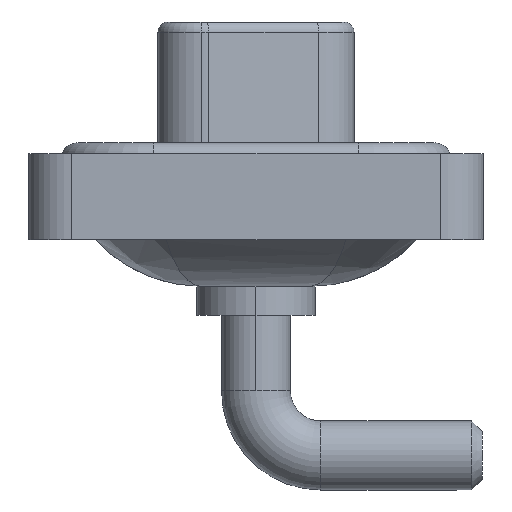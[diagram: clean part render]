
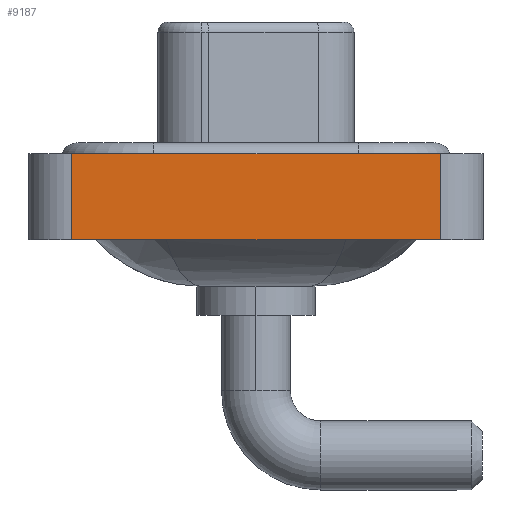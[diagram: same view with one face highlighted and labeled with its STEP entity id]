
A CAD part, left-side view. The second image highlights one B-rep face of the part: STEP entity #9187.
In plain terms, the highlighted planar face has unit normal (-1, 0, 0).
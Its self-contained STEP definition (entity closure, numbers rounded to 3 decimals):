
#529 = LINE ( 'NONE', #6044, #8620 ) ;
#752 = LINE ( 'NONE', #3552, #8677 ) ;
#772 = CARTESIAN_POINT ( 'NONE',  ( -7.25, -8.55, -3.6 ) ) ;
#1699 = DIRECTION ( 'NONE',  ( 0., 0., 1. ) ) ;
#3101 = EDGE_CURVE ( 'NONE', #4943, #15318, #8791, .T. ) ;
#3334 = EDGE_LOOP ( 'NONE', ( #13790, #8606, #15632, #10065 ) ) ;
#3552 = CARTESIAN_POINT ( 'NONE',  ( -7.25, -8.55, 0.4 ) ) ;
#3571 = DIRECTION ( 'NONE',  ( 0., 0., 1. ) ) ;
#3904 = EDGE_CURVE ( 'NONE', #5963, #14046, #752, .T. ) ;
#3946 = PLANE ( 'NONE',  #9314 ) ;
#4545 = CARTESIAN_POINT ( 'NONE',  ( -7.25, -8.55, -3.6 ) ) ;
#4726 = DIRECTION ( 'NONE',  ( 0., -1., 0. ) ) ;
#4943 = VERTEX_POINT ( 'NONE', #11715 ) ;
#5144 = CARTESIAN_POINT ( 'NONE',  ( -7.25, 8.55, 0.4 ) ) ;
#5206 = CARTESIAN_POINT ( 'NONE',  ( -7.25, -8.55, -3.6 ) ) ;
#5963 = VERTEX_POINT ( 'NONE', #5144 ) ;
#6044 = CARTESIAN_POINT ( 'NONE',  ( -7.25, 8.55, -3.6 ) ) ;
#6373 = LINE ( 'NONE', #772, #9791 ) ;
#7018 = CARTESIAN_POINT ( 'NONE',  ( -7.25, -8.55, 0.4 ) ) ;
#7946 = FACE_OUTER_BOUND ( 'NONE', #3334, .T. ) ;
#8131 = DIRECTION ( 'NONE',  ( 0., 0., 1. ) ) ;
#8606 = ORIENTED_EDGE ( 'NONE', *, *, #3904, .F. ) ;
#8620 = VECTOR ( 'NONE', #1699, 1000. ) ;
#8677 = VECTOR ( 'NONE', #4726, 1000. ) ;
#8791 = LINE ( 'NONE', #9385, #17026 ) ;
#9187 = ADVANCED_FACE ( 'NONE', ( #7946 ), #3946, .T. ) ;
#9314 = AXIS2_PLACEMENT_3D ( 'NONE', #5206, #10580, #8131 ) ;
#9385 = CARTESIAN_POINT ( 'NONE',  ( -7.25, -8.55, -3.6 ) ) ;
#9791 = VECTOR ( 'NONE', #3571, 1000. ) ;
#10065 = ORIENTED_EDGE ( 'NONE', *, *, #3101, .T. ) ;
#10580 = DIRECTION ( 'NONE',  ( -1., 0., 0. ) ) ;
#11195 = EDGE_CURVE ( 'NONE', #4943, #5963, #529, .T. ) ;
#11715 = CARTESIAN_POINT ( 'NONE',  ( -7.25, 8.55, -3.6 ) ) ;
#13790 = ORIENTED_EDGE ( 'NONE', *, *, #17811, .T. ) ;
#14046 = VERTEX_POINT ( 'NONE', #7018 ) ;
#15318 = VERTEX_POINT ( 'NONE', #4545 ) ;
#15632 = ORIENTED_EDGE ( 'NONE', *, *, #11195, .F. ) ;
#15889 = DIRECTION ( 'NONE',  ( 0., -1., 0. ) ) ;
#17026 = VECTOR ( 'NONE', #15889, 1000. ) ;
#17811 = EDGE_CURVE ( 'NONE', #15318, #14046, #6373, .T. ) ;
